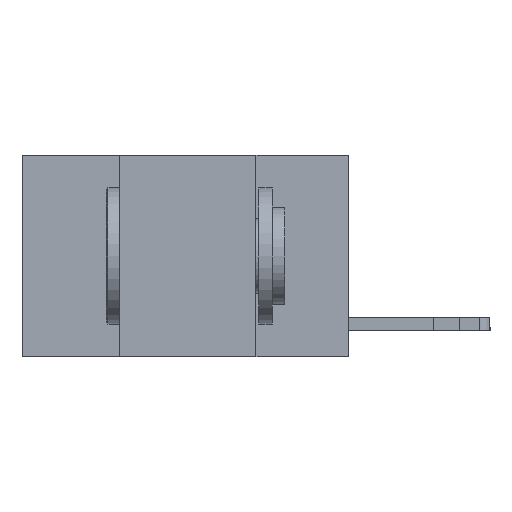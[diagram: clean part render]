
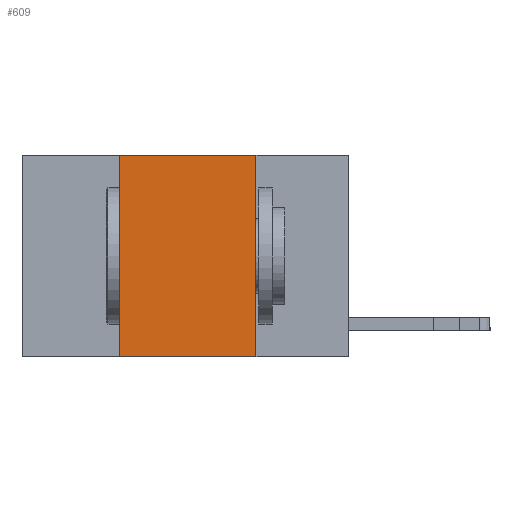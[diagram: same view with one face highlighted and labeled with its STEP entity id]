
A CAD part, left-side view. The second image highlights one B-rep face of the part: STEP entity #609.
In plain terms, the highlighted planar face has unit normal (-1, 0, 0).
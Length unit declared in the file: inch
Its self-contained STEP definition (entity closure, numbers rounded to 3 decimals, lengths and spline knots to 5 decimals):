
#133 = DIRECTION ( 'NONE',  ( 0., 0., -1. ) ) ;
#440 = EDGE_LOOP ( 'NONE', ( #3744, #3384, #3363, #1945 ) ) ;
#520 = VECTOR ( 'NONE', #4965, 39.37008 ) ;
#558 = CARTESIAN_POINT ( 'NONE',  ( 0., 0.17, -0.37 ) ) ;
#609 = ADVANCED_FACE ( 'NONE', ( #3409 ), #12100, .F. ) ;
#1366 = AXIS2_PLACEMENT_3D ( 'NONE', #9932, #4395, #133 ) ;
#1651 = EDGE_CURVE ( 'NONE', #12297, #13284, #2874, .T. ) ;
#1945 = ORIENTED_EDGE ( 'NONE', *, *, #8106, .T. ) ;
#2723 = DIRECTION ( 'NONE',  ( 0., 0., -1. ) ) ;
#2874 = LINE ( 'NONE', #13470, #9865 ) ;
#3363 = ORIENTED_EDGE ( 'NONE', *, *, #13776, .F. ) ;
#3384 = ORIENTED_EDGE ( 'NONE', *, *, #9607, .F. ) ;
#3409 = FACE_OUTER_BOUND ( 'NONE', #440, .T. ) ;
#3744 = ORIENTED_EDGE ( 'NONE', *, *, #1651, .F. ) ;
#3786 = CARTESIAN_POINT ( 'NONE',  ( 0., 0.42, 0. ) ) ;
#3807 = LINE ( 'NONE', #8171, #4898 ) ;
#3814 = LINE ( 'NONE', #5870, #13541 ) ;
#4304 = CARTESIAN_POINT ( 'NONE',  ( 0., 0.17, 0. ) ) ;
#4395 = DIRECTION ( 'NONE',  ( 1., 0., 0. ) ) ;
#4898 = VECTOR ( 'NONE', #12587, 39.37008 ) ;
#4965 = DIRECTION ( 'NONE',  ( 0., -1., 0. ) ) ;
#5870 = CARTESIAN_POINT ( 'NONE',  ( 0., 0.6, -0.37 ) ) ;
#6117 = LINE ( 'NONE', #10514, #520 ) ;
#8106 = EDGE_CURVE ( 'NONE', #12489, #13284, #3814, .T. ) ;
#8171 = CARTESIAN_POINT ( 'NONE',  ( 0., 0.42, 0. ) ) ;
#8446 = CARTESIAN_POINT ( 'NONE',  ( 0., 0.42, -0.37 ) ) ;
#9007 = VERTEX_POINT ( 'NONE', #3786 ) ;
#9607 = EDGE_CURVE ( 'NONE', #9007, #12297, #6117, .T. ) ;
#9865 = VECTOR ( 'NONE', #2723, 39.37008 ) ;
#9932 = CARTESIAN_POINT ( 'NONE',  ( 0., 0.6, 0. ) ) ;
#10514 = CARTESIAN_POINT ( 'NONE',  ( 0., 0.6, 0. ) ) ;
#12100 = PLANE ( 'NONE',  #1366 ) ;
#12297 = VERTEX_POINT ( 'NONE', #4304 ) ;
#12489 = VERTEX_POINT ( 'NONE', #8446 ) ;
#12587 = DIRECTION ( 'NONE',  ( 0., 0., 1. ) ) ;
#13284 = VERTEX_POINT ( 'NONE', #558 ) ;
#13470 = CARTESIAN_POINT ( 'NONE',  ( 0., 0.17, 0. ) ) ;
#13541 = VECTOR ( 'NONE', #13724, 39.37008 ) ;
#13724 = DIRECTION ( 'NONE',  ( 0., -1., 0. ) ) ;
#13776 = EDGE_CURVE ( 'NONE', #12489, #9007, #3807, .T. ) ;
